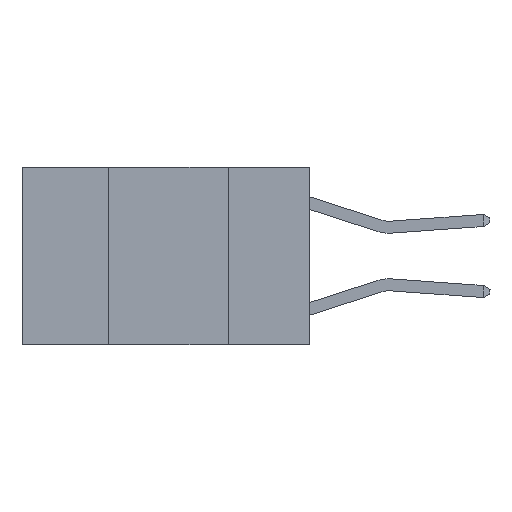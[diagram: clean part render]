
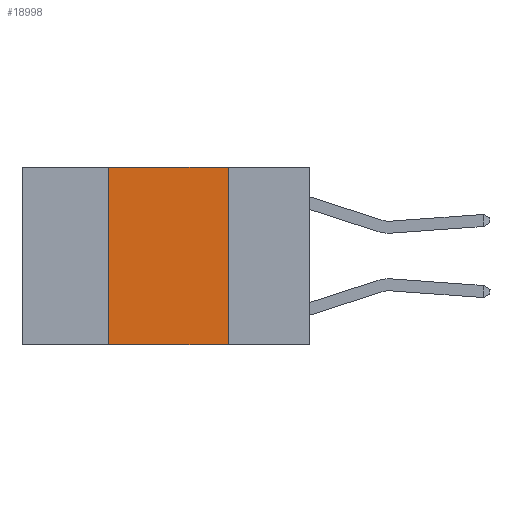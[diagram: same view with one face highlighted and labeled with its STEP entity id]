
A CAD part, left-side view. The second image highlights one B-rep face of the part: STEP entity #18998.
In plain terms, the highlighted planar face has unit normal (-1, 0, 0).
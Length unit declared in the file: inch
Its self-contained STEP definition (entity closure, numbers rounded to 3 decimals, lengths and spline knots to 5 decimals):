
#998 = CARTESIAN_POINT ( 'NONE',  ( 0., 0.6, -0.37 ) ) ;
#1230 = PLANE ( 'NONE',  #14519 ) ;
#1593 = VERTEX_POINT ( 'NONE', #11448 ) ;
#2754 = LINE ( 'NONE', #17454, #26114 ) ;
#3428 = VECTOR ( 'NONE', #7840, 39.37008 ) ;
#3515 = DIRECTION ( 'NONE',  ( 0., 0., -1. ) ) ;
#3609 = DIRECTION ( 'NONE',  ( 0., 0., -1. ) ) ;
#3774 = VERTEX_POINT ( 'NONE', #23390 ) ;
#3885 = CARTESIAN_POINT ( 'NONE',  ( 0., 0.42, -0.37 ) ) ;
#3901 = ORIENTED_EDGE ( 'NONE', *, *, #18410, .F. ) ;
#5754 = LINE ( 'NONE', #8191, #23093 ) ;
#6722 = VERTEX_POINT ( 'NONE', #3885 ) ;
#6879 = DIRECTION ( 'NONE',  ( 0., -1., 0. ) ) ;
#7840 = DIRECTION ( 'NONE',  ( 0., -1., 0. ) ) ;
#8191 = CARTESIAN_POINT ( 'NONE',  ( 0., 0.17, 0. ) ) ;
#9270 = EDGE_CURVE ( 'NONE', #11570, #3774, #5754, .T. ) ;
#9473 = LINE ( 'NONE', #998, #3428 ) ;
#10297 = CARTESIAN_POINT ( 'NONE',  ( 0., 0.6, 0. ) ) ;
#10935 = LINE ( 'NONE', #20483, #22919 ) ;
#11045 = ORIENTED_EDGE ( 'NONE', *, *, #9270, .F. ) ;
#11448 = CARTESIAN_POINT ( 'NONE',  ( 0., 0.42, 0. ) ) ;
#11570 = VERTEX_POINT ( 'NONE', #17166 ) ;
#12894 = DIRECTION ( 'NONE',  ( 0., 0., 1. ) ) ;
#13160 = ORIENTED_EDGE ( 'NONE', *, *, #24302, .F. ) ;
#14016 = EDGE_LOOP ( 'NONE', ( #11045, #13160, #3901, #27920 ) ) ;
#14519 = AXIS2_PLACEMENT_3D ( 'NONE', #10297, #17143, #3515 ) ;
#17143 = DIRECTION ( 'NONE',  ( 1., 0., 0. ) ) ;
#17166 = CARTESIAN_POINT ( 'NONE',  ( 0., 0.17, 0. ) ) ;
#17454 = CARTESIAN_POINT ( 'NONE',  ( 0., 0.42, 0. ) ) ;
#18410 = EDGE_CURVE ( 'NONE', #6722, #1593, #2754, .T. ) ;
#18998 = ADVANCED_FACE ( 'NONE', ( #21875 ), #1230, .F. ) ;
#20483 = CARTESIAN_POINT ( 'NONE',  ( 0., 0.6, 0. ) ) ;
#21875 = FACE_OUTER_BOUND ( 'NONE', #14016, .T. ) ;
#22919 = VECTOR ( 'NONE', #6879, 39.37008 ) ;
#23093 = VECTOR ( 'NONE', #3609, 39.37008 ) ;
#23390 = CARTESIAN_POINT ( 'NONE',  ( 0., 0.17, -0.37 ) ) ;
#24302 = EDGE_CURVE ( 'NONE', #1593, #11570, #10935, .T. ) ;
#26114 = VECTOR ( 'NONE', #12894, 39.37008 ) ;
#27920 = ORIENTED_EDGE ( 'NONE', *, *, #28878, .T. ) ;
#28878 = EDGE_CURVE ( 'NONE', #6722, #3774, #9473, .T. ) ;
